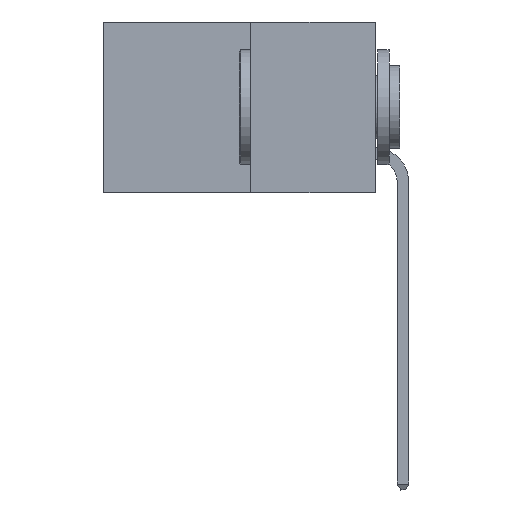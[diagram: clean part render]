
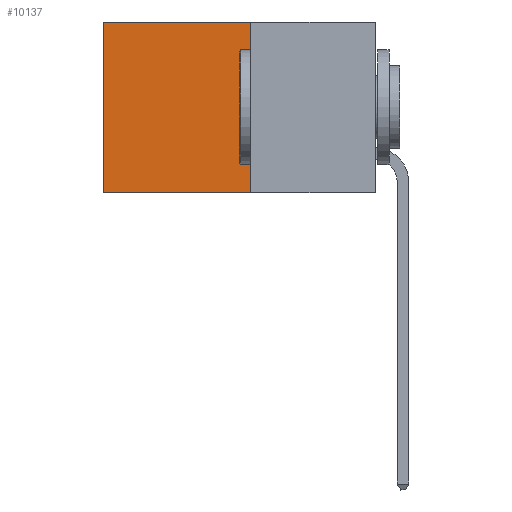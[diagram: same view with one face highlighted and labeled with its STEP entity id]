
A CAD part, left-side view. The second image highlights one B-rep face of the part: STEP entity #10137.
In plain terms, the highlighted planar face has unit normal (-1, 0, 0).
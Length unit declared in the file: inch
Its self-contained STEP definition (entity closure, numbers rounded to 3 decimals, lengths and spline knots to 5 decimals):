
#96 = ORIENTED_EDGE ( 'NONE', *, *, #15912, .F. ) ;
#106 = EDGE_LOOP ( 'NONE', ( #20338, #96, #6410, #19447 ) ) ;
#1251 = VECTOR ( 'NONE', #9941, 39.37008 ) ;
#3080 = CARTESIAN_POINT ( 'NONE',  ( 0.277, 0.59, 0. ) ) ;
#4595 = CARTESIAN_POINT ( 'NONE',  ( 0.277, 0.27, 0. ) ) ;
#5191 = CARTESIAN_POINT ( 'NONE',  ( 0.277, 0.59, -0.37 ) ) ;
#5510 = FACE_OUTER_BOUND ( 'NONE', #106, .T. ) ;
#6230 = EDGE_CURVE ( 'NONE', #17991, #8319, #21511, .T. ) ;
#6410 = ORIENTED_EDGE ( 'NONE', *, *, #6230, .F. ) ;
#6682 = CARTESIAN_POINT ( 'NONE',  ( 0.277, 0.27, -0.37 ) ) ;
#6810 = VERTEX_POINT ( 'NONE', #3080 ) ;
#7200 = CARTESIAN_POINT ( 'NONE',  ( 0.277, 0.27, 0. ) ) ;
#7761 = VECTOR ( 'NONE', #19021, 39.37008 ) ;
#7876 = VECTOR ( 'NONE', #13855, 39.37008 ) ;
#8319 = VERTEX_POINT ( 'NONE', #16247 ) ;
#8829 = DIRECTION ( 'NONE',  ( 0., 1., 0. ) ) ;
#9657 = VECTOR ( 'NONE', #8829, 39.37008 ) ;
#9941 = DIRECTION ( 'NONE',  ( 0., 1., 0. ) ) ;
#10137 = ADVANCED_FACE ( 'NONE', ( #5510 ), #17060, .F. ) ;
#10243 = DIRECTION ( 'NONE',  ( 0., 0., -1. ) ) ;
#10877 = VERTEX_POINT ( 'NONE', #17561 ) ;
#11092 = AXIS2_PLACEMENT_3D ( 'NONE', #6682, #20421, #10243 ) ;
#13855 = DIRECTION ( 'NONE',  ( 0., 0., -1. ) ) ;
#14137 = CARTESIAN_POINT ( 'NONE',  ( 0.277, 0.27, -0.37 ) ) ;
#14265 = LINE ( 'NONE', #17764, #9657 ) ;
#15912 = EDGE_CURVE ( 'NONE', #8319, #10877, #14265, .T. ) ;
#16247 = CARTESIAN_POINT ( 'NONE',  ( 0.277, 0.27, -0.37 ) ) ;
#17060 = PLANE ( 'NONE',  #11092 ) ;
#17561 = CARTESIAN_POINT ( 'NONE',  ( 0.277, 0.59, -0.37 ) ) ;
#17764 = CARTESIAN_POINT ( 'NONE',  ( 0.277, 0.27, -0.37 ) ) ;
#17868 = EDGE_CURVE ( 'NONE', #6810, #10877, #21398, .T. ) ;
#17991 = VERTEX_POINT ( 'NONE', #7200 ) ;
#19021 = DIRECTION ( 'NONE',  ( 0., 0., -1. ) ) ;
#19447 = ORIENTED_EDGE ( 'NONE', *, *, #19579, .T. ) ;
#19579 = EDGE_CURVE ( 'NONE', #17991, #6810, #20784, .T. ) ;
#20338 = ORIENTED_EDGE ( 'NONE', *, *, #17868, .T. ) ;
#20421 = DIRECTION ( 'NONE',  ( 1., 0., 0. ) ) ;
#20784 = LINE ( 'NONE', #4595, #1251 ) ;
#21398 = LINE ( 'NONE', #5191, #7761 ) ;
#21511 = LINE ( 'NONE', #14137, #7876 ) ;
